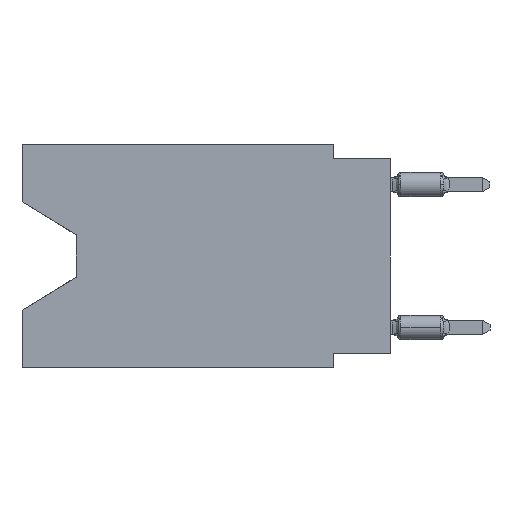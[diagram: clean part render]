
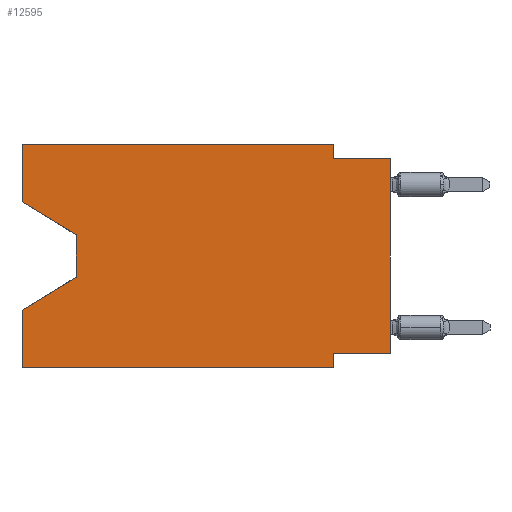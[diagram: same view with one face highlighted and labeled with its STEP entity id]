
A CAD part, left-side view. The second image highlights one B-rep face of the part: STEP entity #12595.
In plain terms, the highlighted planar face has unit normal (-1, 0, 0).
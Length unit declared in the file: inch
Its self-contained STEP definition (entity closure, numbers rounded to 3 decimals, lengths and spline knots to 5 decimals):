
#655 = EDGE_CURVE ( 'NONE', #9364, #3878, #3826, .T. ) ;
#695 = DIRECTION ( 'NONE',  ( 0., 0., -1. ) ) ;
#1210 = LINE ( 'NONE', #5256, #7532 ) ;
#1240 = VERTEX_POINT ( 'NONE', #12413 ) ;
#1318 = CARTESIAN_POINT ( 'NONE',  ( 0., 0.645, 0. ) ) ;
#1500 = DIRECTION ( 'NONE',  ( 0., -0.855, -0.519 ) ) ;
#1704 = VECTOR ( 'NONE', #15805, 39.37008 ) ;
#1843 = EDGE_CURVE ( 'NONE', #2709, #12052, #1210, .T. ) ;
#2098 = CARTESIAN_POINT ( 'NONE',  ( 0., 0.55, -0.158 ) ) ;
#2419 = CARTESIAN_POINT ( 'NONE',  ( 0., 0., -0.365 ) ) ;
#2488 = ORIENTED_EDGE ( 'NONE', *, *, #12762, .T. ) ;
#2709 = VERTEX_POINT ( 'NONE', #6846 ) ;
#2929 = LINE ( 'NONE', #7934, #12881 ) ;
#3122 = ORIENTED_EDGE ( 'NONE', *, *, #3588, .F. ) ;
#3169 = CARTESIAN_POINT ( 'NONE',  ( 0., 0.1, -0.365 ) ) ;
#3588 = EDGE_CURVE ( 'NONE', #9364, #12052, #15484, .T. ) ;
#3826 = LINE ( 'NONE', #4971, #1704 ) ;
#3878 = VERTEX_POINT ( 'NONE', #12295 ) ;
#4221 = VECTOR ( 'NONE', #12378, 39.37008 ) ;
#4272 = CARTESIAN_POINT ( 'NONE',  ( 0., 0., -0.365 ) ) ;
#4300 = CARTESIAN_POINT ( 'NONE',  ( 0., 0.1, 0. ) ) ;
#4416 = EDGE_CURVE ( 'NONE', #13330, #11067, #11215, .T. ) ;
#4581 = DIRECTION ( 'NONE',  ( 1., 0., 0. ) ) ;
#4971 = CARTESIAN_POINT ( 'NONE',  ( 0., 0.645, -0.39 ) ) ;
#5110 = ORIENTED_EDGE ( 'NONE', *, *, #655, .T. ) ;
#5231 = VERTEX_POINT ( 'NONE', #3169 ) ;
#5256 = CARTESIAN_POINT ( 'NONE',  ( 0., 0.55, -0.232 ) ) ;
#5332 = DIRECTION ( 'NONE',  ( 0., 0., 1. ) ) ;
#5413 = DIRECTION ( 'NONE',  ( 0., -1., 0. ) ) ;
#5419 = CARTESIAN_POINT ( 'NONE',  ( 0., 0.645, 0. ) ) ;
#5737 = EDGE_CURVE ( 'NONE', #6900, #5231, #10339, .T. ) ;
#5884 = DIRECTION ( 'NONE',  ( 0., 0., 1. ) ) ;
#5926 = VECTOR ( 'NONE', #17315, 39.37008 ) ;
#6394 = ORIENTED_EDGE ( 'NONE', *, *, #16839, .T. ) ;
#6445 = DIRECTION ( 'NONE',  ( 0., 1., 0. ) ) ;
#6649 = CARTESIAN_POINT ( 'NONE',  ( 0., 0., 0. ) ) ;
#6718 = VECTOR ( 'NONE', #5332, 39.37008 ) ;
#6750 = ORIENTED_EDGE ( 'NONE', *, *, #8394, .F. ) ;
#6846 = CARTESIAN_POINT ( 'NONE',  ( 0., 0.55, -0.232 ) ) ;
#6900 = VERTEX_POINT ( 'NONE', #4272 ) ;
#7024 = VECTOR ( 'NONE', #5884, 39.37008 ) ;
#7315 = ORIENTED_EDGE ( 'NONE', *, *, #10758, .F. ) ;
#7504 = LINE ( 'NONE', #9103, #13087 ) ;
#7532 = VECTOR ( 'NONE', #16083, 39.37008 ) ;
#7741 = VECTOR ( 'NONE', #5413, 39.37008 ) ;
#7934 = CARTESIAN_POINT ( 'NONE',  ( 0., 0.1, -0.39 ) ) ;
#7950 = LINE ( 'NONE', #13587, #7741 ) ;
#8280 = DIRECTION ( 'NONE',  ( 0., 0., -1. ) ) ;
#8394 = EDGE_CURVE ( 'NONE', #5231, #3878, #2929, .T. ) ;
#8587 = LINE ( 'NONE', #15111, #4221 ) ;
#8642 = VECTOR ( 'NONE', #1500, 39.37008 ) ;
#8785 = CARTESIAN_POINT ( 'NONE',  ( 0., 0.645, 0. ) ) ;
#9103 = CARTESIAN_POINT ( 'NONE',  ( 0., 0.55, -0.158 ) ) ;
#9289 = LINE ( 'NONE', #5419, #6718 ) ;
#9364 = VERTEX_POINT ( 'NONE', #12284 ) ;
#10104 = FACE_OUTER_BOUND ( 'NONE', #16198, .T. ) ;
#10339 = LINE ( 'NONE', #2419, #16862 ) ;
#10542 = LINE ( 'NONE', #6649, #5926 ) ;
#10758 = EDGE_CURVE ( 'NONE', #1240, #12233, #9289, .T. ) ;
#10794 = ORIENTED_EDGE ( 'NONE', *, *, #5737, .F. ) ;
#11067 = VERTEX_POINT ( 'NONE', #13433 ) ;
#11104 = EDGE_CURVE ( 'NONE', #11126, #13330, #8587, .T. ) ;
#11126 = VERTEX_POINT ( 'NONE', #4300 ) ;
#11215 = LINE ( 'NONE', #13383, #12950 ) ;
#11838 = AXIS2_PLACEMENT_3D ( 'NONE', #12738, #4581, #695 ) ;
#11977 = ORIENTED_EDGE ( 'NONE', *, *, #13645, .T. ) ;
#12052 = VERTEX_POINT ( 'NONE', #12243 ) ;
#12233 = VERTEX_POINT ( 'NONE', #1318 ) ;
#12243 = CARTESIAN_POINT ( 'NONE',  ( 0., 0.645, -0.28975 ) ) ;
#12284 = CARTESIAN_POINT ( 'NONE',  ( 0., 0.645, -0.39 ) ) ;
#12295 = CARTESIAN_POINT ( 'NONE',  ( 0., 0.1, -0.39 ) ) ;
#12378 = DIRECTION ( 'NONE',  ( 0., 0., -1. ) ) ;
#12407 = CARTESIAN_POINT ( 'NONE',  ( 0., 0.645, -0.10025 ) ) ;
#12413 = CARTESIAN_POINT ( 'NONE',  ( 0., 0.645, -0.10025 ) ) ;
#12563 = VERTEX_POINT ( 'NONE', #2098 ) ;
#12586 = CARTESIAN_POINT ( 'NONE',  ( 0., 0.1, -0.025 ) ) ;
#12595 = ADVANCED_FACE ( 'NONE', ( #10104 ), #13893, .F. ) ;
#12738 = CARTESIAN_POINT ( 'NONE',  ( 0., 0.645, 0. ) ) ;
#12762 = EDGE_CURVE ( 'NONE', #6900, #11067, #10542, .T. ) ;
#12881 = VECTOR ( 'NONE', #8280, 39.37008 ) ;
#12950 = VECTOR ( 'NONE', #13300, 39.37008 ) ;
#12982 = DIRECTION ( 'NONE',  ( 0., 0., -1. ) ) ;
#13087 = VECTOR ( 'NONE', #12982, 39.37008 ) ;
#13300 = DIRECTION ( 'NONE',  ( 0., -1., 0. ) ) ;
#13330 = VERTEX_POINT ( 'NONE', #12586 ) ;
#13383 = CARTESIAN_POINT ( 'NONE',  ( 0., 0., -0.025 ) ) ;
#13433 = CARTESIAN_POINT ( 'NONE',  ( 0., 0., -0.025 ) ) ;
#13587 = CARTESIAN_POINT ( 'NONE',  ( 0., 0.645, 0. ) ) ;
#13645 = EDGE_CURVE ( 'NONE', #1240, #12563, #16367, .T. ) ;
#13749 = ORIENTED_EDGE ( 'NONE', *, *, #16902, .F. ) ;
#13893 = PLANE ( 'NONE',  #11838 ) ;
#14475 = ORIENTED_EDGE ( 'NONE', *, *, #4416, .F. ) ;
#14947 = ORIENTED_EDGE ( 'NONE', *, *, #11104, .F. ) ;
#15111 = CARTESIAN_POINT ( 'NONE',  ( 0., 0.1, 0. ) ) ;
#15484 = LINE ( 'NONE', #8785, #7024 ) ;
#15805 = DIRECTION ( 'NONE',  ( 0., -1., 0. ) ) ;
#15813 = ORIENTED_EDGE ( 'NONE', *, *, #1843, .T. ) ;
#16083 = DIRECTION ( 'NONE',  ( 0., 0.855, -0.519 ) ) ;
#16198 = EDGE_LOOP ( 'NONE', ( #11977, #6394, #15813, #3122, #5110, #6750, #10794, #2488, #14475, #14947, #13749, #7315 ) ) ;
#16367 = LINE ( 'NONE', #12407, #8642 ) ;
#16839 = EDGE_CURVE ( 'NONE', #12563, #2709, #7504, .T. ) ;
#16862 = VECTOR ( 'NONE', #6445, 39.37008 ) ;
#16902 = EDGE_CURVE ( 'NONE', #12233, #11126, #7950, .T. ) ;
#17315 = DIRECTION ( 'NONE',  ( 0., 0., 1. ) ) ;
